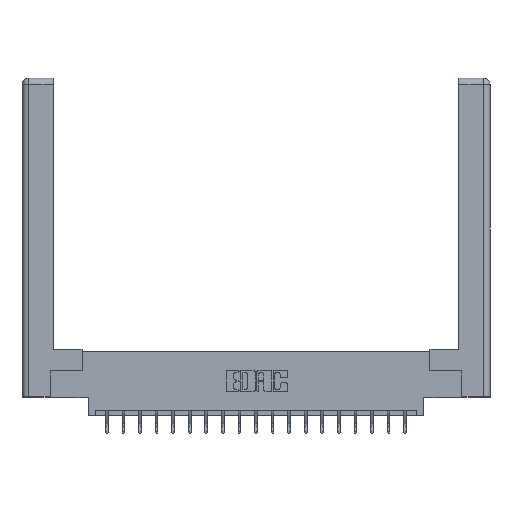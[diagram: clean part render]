
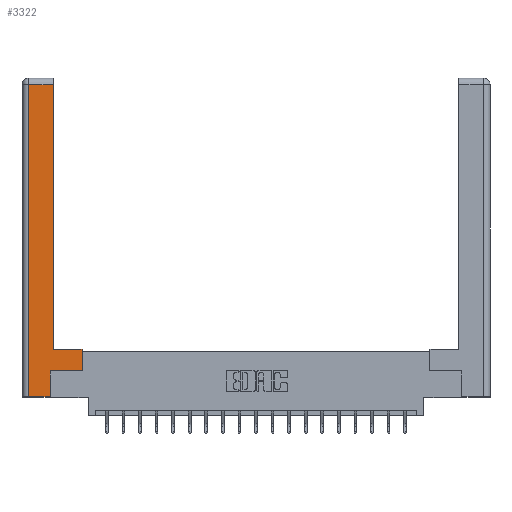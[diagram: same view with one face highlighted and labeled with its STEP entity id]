
A CAD part, top view. The second image highlights one B-rep face of the part: STEP entity #3322.
In plain terms, the highlighted planar face has unit normal (0, 0, 1).
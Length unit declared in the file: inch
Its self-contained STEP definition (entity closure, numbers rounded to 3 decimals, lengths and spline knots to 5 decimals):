
#27 = LINE ( 'NONE', #2078, #11275 ) ;
#372 = ORIENTED_EDGE ( 'NONE', *, *, #13346, .T. ) ;
#549 = EDGE_CURVE ( 'NONE', #18518, #12632, #7749, .T. ) ;
#649 = LINE ( 'NONE', #15898, #18893 ) ;
#693 = VECTOR ( 'NONE', #9957, 39.37008 ) ;
#959 = LINE ( 'NONE', #19605, #693 ) ;
#1022 = LINE ( 'NONE', #9672, #15026 ) ;
#1155 = EDGE_LOOP ( 'NONE', ( #372, #16111, #12447, #3074, #11554, #11805, #9520, #19923 ) ) ;
#1195 = CARTESIAN_POINT ( 'NONE',  ( 0.0615, 2.94, 0. ) ) ;
#1623 = EDGE_CURVE ( 'NONE', #12632, #18025, #959, .T. ) ;
#2078 = CARTESIAN_POINT ( 'NONE',  ( 0.295, 0.45, 0. ) ) ;
#2263 = CARTESIAN_POINT ( 'NONE',  ( 0.295, 3., 0. ) ) ;
#2310 = EDGE_CURVE ( 'NONE', #19024, #15130, #14658, .T. ) ;
#2518 = EDGE_CURVE ( 'NONE', #18025, #20318, #649, .T. ) ;
#2849 = CARTESIAN_POINT ( 'NONE',  ( 0.265, 0., 0. ) ) ;
#2892 = DIRECTION ( 'NONE',  ( -1., 0., 0. ) ) ;
#3074 = ORIENTED_EDGE ( 'NONE', *, *, #2518, .T. ) ;
#3322 = ADVANCED_FACE ( 'NONE', ( #5663 ), #8160, .F. ) ;
#4072 = AXIS2_PLACEMENT_3D ( 'NONE', #12962, #12811, #4895 ) ;
#4273 = CARTESIAN_POINT ( 'NONE',  ( 0.295, 2.94, 0. ) ) ;
#4452 = CARTESIAN_POINT ( 'NONE',  ( 0.265, 0.245, 0. ) ) ;
#4869 = DIRECTION ( 'NONE',  ( 0., 1., 0. ) ) ;
#4895 = DIRECTION ( 'NONE',  ( -1., 0., 0. ) ) ;
#5563 = EDGE_CURVE ( 'NONE', #20318, #19024, #12194, .T. ) ;
#5663 = FACE_OUTER_BOUND ( 'NONE', #1155, .T. ) ;
#5882 = LINE ( 'NONE', #2263, #19623 ) ;
#6284 = CARTESIAN_POINT ( 'NONE',  ( 0.295, 0.45, 0. ) ) ;
#7489 = VECTOR ( 'NONE', #2892, 39.37008 ) ;
#7749 = LINE ( 'NONE', #1195, #7489 ) ;
#8160 = PLANE ( 'NONE',  #4072 ) ;
#8415 = VECTOR ( 'NONE', #16784, 39.37008 ) ;
#8581 = CARTESIAN_POINT ( 'NONE',  ( 0.0615, 2.94, 0. ) ) ;
#9520 = ORIENTED_EDGE ( 'NONE', *, *, #15111, .T. ) ;
#9672 = CARTESIAN_POINT ( 'NONE',  ( 0.565, 0.45, 0. ) ) ;
#9957 = DIRECTION ( 'NONE',  ( 0., -1., 0. ) ) ;
#11248 = CARTESIAN_POINT ( 'NONE',  ( 0.565, 0.45, 0. ) ) ;
#11275 = VECTOR ( 'NONE', #13223, 39.37008 ) ;
#11554 = ORIENTED_EDGE ( 'NONE', *, *, #5563, .T. ) ;
#11805 = ORIENTED_EDGE ( 'NONE', *, *, #2310, .T. ) ;
#11972 = CARTESIAN_POINT ( 'NONE',  ( 0.565, 0.245, 0. ) ) ;
#12194 = LINE ( 'NONE', #4452, #18459 ) ;
#12447 = ORIENTED_EDGE ( 'NONE', *, *, #1623, .T. ) ;
#12632 = VERTEX_POINT ( 'NONE', #8581 ) ;
#12759 = DIRECTION ( 'NONE',  ( 1., 0., 0. ) ) ;
#12811 = DIRECTION ( 'NONE',  ( 0., 0., -1. ) ) ;
#12962 = CARTESIAN_POINT ( 'NONE',  ( 0., 0., 0. ) ) ;
#13223 = DIRECTION ( 'NONE',  ( -1., 0., 0. ) ) ;
#13346 = EDGE_CURVE ( 'NONE', #14584, #18518, #5882, .T. ) ;
#13857 = DIRECTION ( 'NONE',  ( 0., 1., 0. ) ) ;
#14050 = VERTEX_POINT ( 'NONE', #11248 ) ;
#14117 = CARTESIAN_POINT ( 'NONE',  ( 0.565, 0.245, 0. ) ) ;
#14584 = VERTEX_POINT ( 'NONE', #6284 ) ;
#14658 = LINE ( 'NONE', #11972, #8415 ) ;
#15026 = VECTOR ( 'NONE', #4869, 39.37008 ) ;
#15111 = EDGE_CURVE ( 'NONE', #15130, #14050, #1022, .T. ) ;
#15130 = VERTEX_POINT ( 'NONE', #14117 ) ;
#15474 = EDGE_CURVE ( 'NONE', #14050, #14584, #27, .T. ) ;
#15563 = DIRECTION ( 'NONE',  ( 0., 1., 0. ) ) ;
#15898 = CARTESIAN_POINT ( 'NONE',  ( 0.265, 0., 0. ) ) ;
#16111 = ORIENTED_EDGE ( 'NONE', *, *, #549, .T. ) ;
#16784 = DIRECTION ( 'NONE',  ( 1., 0., 0. ) ) ;
#16855 = CARTESIAN_POINT ( 'NONE',  ( 0.265, 0.245, 0. ) ) ;
#18025 = VERTEX_POINT ( 'NONE', #18998 ) ;
#18459 = VECTOR ( 'NONE', #15563, 39.37008 ) ;
#18518 = VERTEX_POINT ( 'NONE', #4273 ) ;
#18893 = VECTOR ( 'NONE', #12759, 39.37008 ) ;
#18998 = CARTESIAN_POINT ( 'NONE',  ( 0.0615, 0., 0. ) ) ;
#19024 = VERTEX_POINT ( 'NONE', #16855 ) ;
#19605 = CARTESIAN_POINT ( 'NONE',  ( 0.0615, 0., 0. ) ) ;
#19623 = VECTOR ( 'NONE', #13857, 39.37008 ) ;
#19923 = ORIENTED_EDGE ( 'NONE', *, *, #15474, .T. ) ;
#20318 = VERTEX_POINT ( 'NONE', #2849 ) ;
